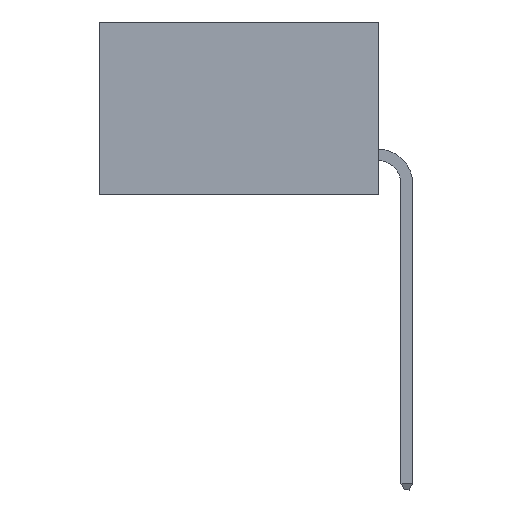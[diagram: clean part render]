
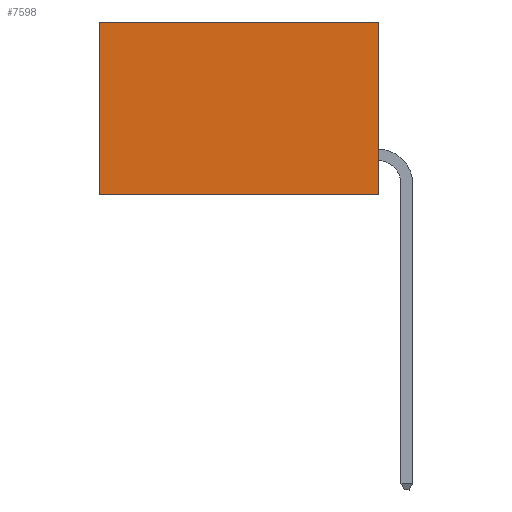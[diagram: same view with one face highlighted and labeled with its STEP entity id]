
A CAD part, left-side view. The second image highlights one B-rep face of the part: STEP entity #7598.
In plain terms, the highlighted planar face has unit normal (-1, 0, 0).
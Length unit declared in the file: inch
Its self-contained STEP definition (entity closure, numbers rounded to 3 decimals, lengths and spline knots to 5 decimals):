
#360 = CARTESIAN_POINT ( 'NONE',  ( 0.2615, 0.6, 0. ) ) ;
#470 = CARTESIAN_POINT ( 'NONE',  ( 0.2615, 0., -0.37 ) ) ;
#909 = EDGE_CURVE ( 'NONE', #13421, #10844, #2795, .T. ) ;
#1726 = DIRECTION ( 'NONE',  ( 0., 0., -1. ) ) ;
#2517 = CARTESIAN_POINT ( 'NONE',  ( 0.2615, 0., 0. ) ) ;
#2795 = LINE ( 'NONE', #7688, #5541 ) ;
#2809 = PLANE ( 'NONE',  #9856 ) ;
#3108 = LINE ( 'NONE', #11636, #11156 ) ;
#3832 = LINE ( 'NONE', #13334, #8067 ) ;
#4078 = VECTOR ( 'NONE', #8114, 39.37008 ) ;
#4100 = DIRECTION ( 'NONE',  ( 0., 1., 0. ) ) ;
#4858 = CARTESIAN_POINT ( 'NONE',  ( 0.2615, 0., -0.37 ) ) ;
#5186 = EDGE_CURVE ( 'NONE', #6566, #13536, #3108, .T. ) ;
#5541 = VECTOR ( 'NONE', #6971, 39.37008 ) ;
#6566 = VERTEX_POINT ( 'NONE', #2517 ) ;
#6971 = DIRECTION ( 'NONE',  ( 0., 1., 0. ) ) ;
#7114 = DIRECTION ( 'NONE',  ( 1., 0., 0. ) ) ;
#7598 = ADVANCED_FACE ( 'NONE', ( #12459 ), #2809, .F. ) ;
#7688 = CARTESIAN_POINT ( 'NONE',  ( 0.2615, 0., -0.37 ) ) ;
#7778 = CARTESIAN_POINT ( 'NONE',  ( 0.2615, 0.6, -0.37 ) ) ;
#8067 = VECTOR ( 'NONE', #1726, 39.37008 ) ;
#8114 = DIRECTION ( 'NONE',  ( 0., 0., -1. ) ) ;
#8255 = EDGE_CURVE ( 'NONE', #13536, #10844, #3832, .T. ) ;
#8672 = ORIENTED_EDGE ( 'NONE', *, *, #8255, .T. ) ;
#9299 = DIRECTION ( 'NONE',  ( 0., 0., -1. ) ) ;
#9569 = EDGE_LOOP ( 'NONE', ( #8672, #11340, #10682, #13872 ) ) ;
#9856 = AXIS2_PLACEMENT_3D ( 'NONE', #470, #7114, #9299 ) ;
#10297 = LINE ( 'NONE', #4858, #4078 ) ;
#10682 = ORIENTED_EDGE ( 'NONE', *, *, #12811, .F. ) ;
#10844 = VERTEX_POINT ( 'NONE', #7778 ) ;
#11156 = VECTOR ( 'NONE', #4100, 39.37008 ) ;
#11340 = ORIENTED_EDGE ( 'NONE', *, *, #909, .F. ) ;
#11636 = CARTESIAN_POINT ( 'NONE',  ( 0.2615, 0., 0. ) ) ;
#12459 = FACE_OUTER_BOUND ( 'NONE', #9569, .T. ) ;
#12811 = EDGE_CURVE ( 'NONE', #6566, #13421, #10297, .T. ) ;
#12914 = CARTESIAN_POINT ( 'NONE',  ( 0.2615, 0., -0.37 ) ) ;
#13334 = CARTESIAN_POINT ( 'NONE',  ( 0.2615, 0.6, -0.37 ) ) ;
#13421 = VERTEX_POINT ( 'NONE', #12914 ) ;
#13536 = VERTEX_POINT ( 'NONE', #360 ) ;
#13872 = ORIENTED_EDGE ( 'NONE', *, *, #5186, .T. ) ;
